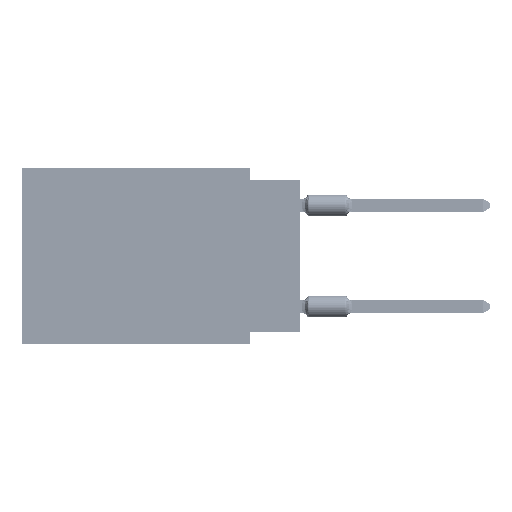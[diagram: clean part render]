
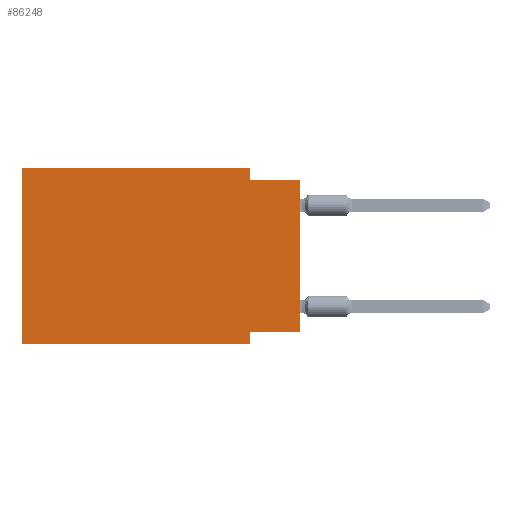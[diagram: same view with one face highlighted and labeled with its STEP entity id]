
A CAD part, left-side view. The second image highlights one B-rep face of the part: STEP entity #86248.
In plain terms, the highlighted planar face has unit normal (-1, 0, 0).
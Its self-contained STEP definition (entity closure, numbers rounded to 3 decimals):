
#2436 = LINE ( 'NONE', #102062, #38473 ) ;
#2467 = EDGE_LOOP ( 'NONE', ( #6026, #108942, #45323, #88498, #54108, #23389, #64026, #74811 ) ) ;
#4492 = PLANE ( 'NONE',  #24570 ) ;
#4725 = EDGE_CURVE ( 'NONE', #60630, #46186, #9277, .T. ) ;
#5317 = CARTESIAN_POINT ( 'NONE',  ( 0., 0., -0.635 ) ) ;
#5390 = CARTESIAN_POINT ( 'NONE',  ( 0., 13.97, 0. ) ) ;
#6026 = ORIENTED_EDGE ( 'NONE', *, *, #87234, .T. ) ;
#6106 = EDGE_CURVE ( 'NONE', #66750, #36846, #72966, .T. ) ;
#6170 = VERTEX_POINT ( 'NONE', #21906 ) ;
#7184 = DIRECTION ( 'NONE',  ( 0., -1., 0. ) ) ;
#7463 = DIRECTION ( 'NONE',  ( 0., 0., -1. ) ) ;
#9277 = LINE ( 'NONE', #74642, #11759 ) ;
#11135 = LINE ( 'NONE', #30879, #41649 ) ;
#11176 = DIRECTION ( 'NONE',  ( 0., 0., 1. ) ) ;
#11738 = EDGE_CURVE ( 'NONE', #86703, #55497, #58776, .T. ) ;
#11759 = VECTOR ( 'NONE', #111230, 1000. ) ;
#13831 = CARTESIAN_POINT ( 'NONE',  ( 0., 2.54, -8.255 ) ) ;
#14948 = CARTESIAN_POINT ( 'NONE',  ( 0., 13.97, 0. ) ) ;
#18686 = CARTESIAN_POINT ( 'NONE',  ( 0., 13.97, -8.89 ) ) ;
#21906 = CARTESIAN_POINT ( 'NONE',  ( 0., 2.54, -8.89 ) ) ;
#23389 = ORIENTED_EDGE ( 'NONE', *, *, #106929, .T. ) ;
#24570 = AXIS2_PLACEMENT_3D ( 'NONE', #115463, #74021, #7463 ) ;
#28685 = VECTOR ( 'NONE', #108965, 1000. ) ;
#30879 = CARTESIAN_POINT ( 'NONE',  ( 0., 0., -0.635 ) ) ;
#30919 = LINE ( 'NONE', #48338, #109110 ) ;
#31708 = CARTESIAN_POINT ( 'NONE',  ( 0., 13.97, 0. ) ) ;
#33692 = DIRECTION ( 'NONE',  ( 0., -1., 0. ) ) ;
#35757 = CARTESIAN_POINT ( 'NONE',  ( 0., 2.54, 0. ) ) ;
#35988 = VECTOR ( 'NONE', #33692, 1000. ) ;
#36846 = VERTEX_POINT ( 'NONE', #36973 ) ;
#36973 = CARTESIAN_POINT ( 'NONE',  ( 0., 2.54, -0.635 ) ) ;
#38473 = VECTOR ( 'NONE', #56469, 1000. ) ;
#41649 = VECTOR ( 'NONE', #103495, 1000. ) ;
#45323 = ORIENTED_EDGE ( 'NONE', *, *, #6106, .F. ) ;
#46186 = VERTEX_POINT ( 'NONE', #13831 ) ;
#48338 = CARTESIAN_POINT ( 'NONE',  ( 0., 0., 0. ) ) ;
#49766 = DIRECTION ( 'NONE',  ( 0., 0., 1. ) ) ;
#50092 = FACE_OUTER_BOUND ( 'NONE', #2467, .T. ) ;
#54108 = ORIENTED_EDGE ( 'NONE', *, *, #11738, .F. ) ;
#55497 = VERTEX_POINT ( 'NONE', #31708 ) ;
#56469 = DIRECTION ( 'NONE',  ( 0., 0., -1. ) ) ;
#57310 = EDGE_CURVE ( 'NONE', #36846, #92338, #11135, .T. ) ;
#58257 = CARTESIAN_POINT ( 'NONE',  ( 0., 0., -8.255 ) ) ;
#58776 = LINE ( 'NONE', #14948, #89669 ) ;
#60630 = VERTEX_POINT ( 'NONE', #58257 ) ;
#63000 = EDGE_CURVE ( 'NONE', #46186, #6170, #2436, .T. ) ;
#64026 = ORIENTED_EDGE ( 'NONE', *, *, #63000, .F. ) ;
#66750 = VERTEX_POINT ( 'NONE', #82272 ) ;
#72966 = LINE ( 'NONE', #35757, #28685 ) ;
#74021 = DIRECTION ( 'NONE',  ( 1., 0., 0. ) ) ;
#74642 = CARTESIAN_POINT ( 'NONE',  ( 0., 0., -8.255 ) ) ;
#74811 = ORIENTED_EDGE ( 'NONE', *, *, #4725, .F. ) ;
#78262 = EDGE_CURVE ( 'NONE', #55497, #66750, #79776, .T. ) ;
#79776 = LINE ( 'NONE', #5390, #93212 ) ;
#82271 = CARTESIAN_POINT ( 'NONE',  ( 0., 13.97, -8.89 ) ) ;
#82272 = CARTESIAN_POINT ( 'NONE',  ( 0., 2.54, 0. ) ) ;
#86248 = ADVANCED_FACE ( 'NONE', ( #50092 ), #4492, .F. ) ;
#86703 = VERTEX_POINT ( 'NONE', #18686 ) ;
#87234 = EDGE_CURVE ( 'NONE', #60630, #92338, #30919, .T. ) ;
#88498 = ORIENTED_EDGE ( 'NONE', *, *, #78262, .F. ) ;
#89669 = VECTOR ( 'NONE', #49766, 1000. ) ;
#92338 = VERTEX_POINT ( 'NONE', #5317 ) ;
#93212 = VECTOR ( 'NONE', #7184, 1000. ) ;
#102062 = CARTESIAN_POINT ( 'NONE',  ( 0., 2.54, -8.89 ) ) ;
#103495 = DIRECTION ( 'NONE',  ( 0., -1., 0. ) ) ;
#106929 = EDGE_CURVE ( 'NONE', #86703, #6170, #109272, .T. ) ;
#108942 = ORIENTED_EDGE ( 'NONE', *, *, #57310, .F. ) ;
#108965 = DIRECTION ( 'NONE',  ( 0., 0., -1. ) ) ;
#109110 = VECTOR ( 'NONE', #11176, 1000. ) ;
#109272 = LINE ( 'NONE', #82271, #35988 ) ;
#111230 = DIRECTION ( 'NONE',  ( 0., 1., 0. ) ) ;
#115463 = CARTESIAN_POINT ( 'NONE',  ( 0., 13.97, 0. ) ) ;
